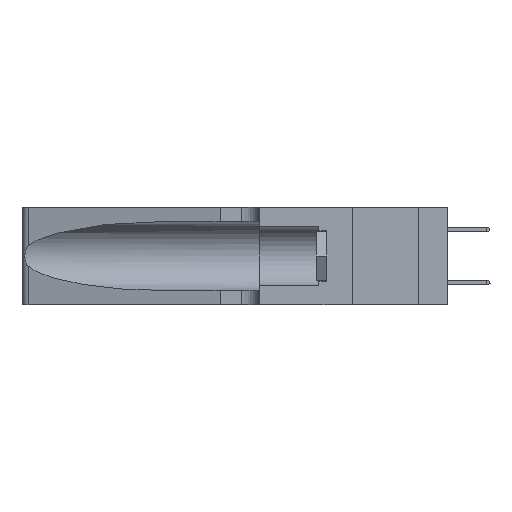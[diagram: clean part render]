
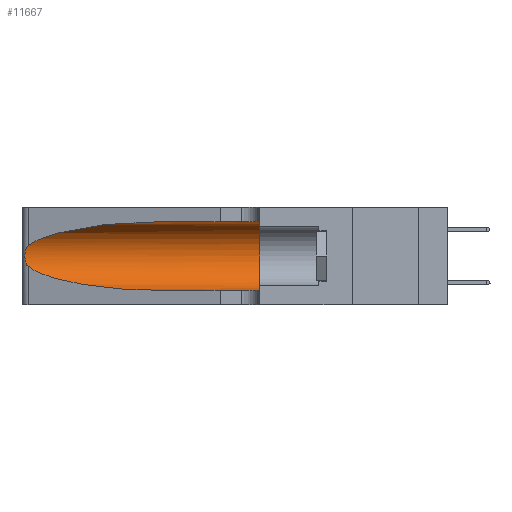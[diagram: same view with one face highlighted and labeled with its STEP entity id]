
A CAD part, left-side view. The second image highlights one B-rep face of the part: STEP entity #11667.
In plain terms, the highlighted cylindrical face has radius 3.308 mm (diameter 6.617 mm), a partial arc.
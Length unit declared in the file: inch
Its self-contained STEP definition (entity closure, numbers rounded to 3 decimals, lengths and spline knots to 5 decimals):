
#311 = VERTEX_POINT ( 'NONE', #428 ) ;
#428 = CARTESIAN_POINT ( 'NONE',  ( 0.1305, 0.72297, 0.05475 ) ) ;
#748 = CARTESIAN_POINT ( 'NONE',  ( 0.26017, 1.23833, 0.17102 ) ) ;
#1213 =( BOUNDED_CURVE ( )  B_SPLINE_CURVE ( 3, ( #29849, #4670, #22316, #2361 ),
 .UNSPECIFIED., .F., .T. ) 
 B_SPLINE_CURVE_WITH_KNOTS ( ( 4, 4 ),
 ( 1.5708, 2.84003 ),
 .UNSPECIFIED. ) 
 CURVE ( )  GEOMETRIC_REPRESENTATION_ITEM ( )  RATIONAL_B_SPLINE_CURVE ( ( 1., 0.87, 0.87, 1. ) ) 
 REPRESENTATION_ITEM ( '' )  );
#1276 = EDGE_CURVE ( 'NONE', #22835, #1857, #1213, .T. ) ;
#1351 = CYLINDRICAL_SURFACE ( 'NONE', #23014, 0.13025 ) ;
#1857 = VERTEX_POINT ( 'NONE', #15176 ) ;
#2094 = CIRCLE ( 'NONE', #8127, 0.13025 ) ;
#2361 = CARTESIAN_POINT ( 'NONE',  ( 0.25487, 1.22718, 0.22369 ) ) ;
#2456 = DIRECTION ( 'NONE',  ( 0., -1., 0. ) ) ;
#2646 = EDGE_CURVE ( 'NONE', #1857, #17677, #9089, .T. ) ;
#3270 = CARTESIAN_POINT ( 'NONE',  ( 0.26075, 1.23896, 0.19203 ) ) ;
#3482 = CARTESIAN_POINT ( 'NONE',  ( 0.25555, 1.22994, 0.2215 ) ) ;
#4023 = DIRECTION ( 'NONE',  ( 0., 1., 0. ) ) ;
#4670 = CARTESIAN_POINT ( 'NONE',  ( 0.18966, 0.96281, 0.31525 ) ) ;
#5170 = CARTESIAN_POINT ( 'NONE',  ( 0.18966, 0.96281, 0.05475 ) ) ;
#5290 = ORIENTED_EDGE ( 'NONE', *, *, #2646, .T. ) ;
#5950 = EDGE_CURVE ( 'NONE', #30631, #10290, #2094, .T. ) ;
#6088 = EDGE_CURVE ( 'NONE', #22835, #30631, #28123, .T. ) ;
#6875 = FACE_OUTER_BOUND ( 'NONE', #13525, .T. ) ;
#7807 = EDGE_CURVE ( 'NONE', #17677, #311, #10099, .T. ) ;
#7984 = ORIENTED_EDGE ( 'NONE', *, *, #5950, .F. ) ;
#8127 = AXIS2_PLACEMENT_3D ( 'NONE', #16268, #4023, #18768 ) ;
#8325 = CARTESIAN_POINT ( 'NONE',  ( 0.25487, 1.22718, 0.14631 ) ) ;
#8363 = VECTOR ( 'NONE', #23305, 39.37008 ) ;
#8463 = CARTESIAN_POINT ( 'NONE',  ( 0.25487, 1.22718, 0.14631 ) ) ;
#8469 = ORIENTED_EDGE ( 'NONE', *, *, #26718, .T. ) ;
#9089 = B_SPLINE_CURVE_WITH_KNOTS ( 'NONE', 3,
 ( #13322, #3482, #10686, #26232, #13214, #23803, #3270, #31138, #748, #21122, #23702, #11120, #18343, #8463 ),
 .UNSPECIFIED., .F., .F.,
 ( 4, 2, 2, 2, 2, 2, 4 ),
 ( 0., 0.00027, 0.00053, 0.00107, 0.0016, 0.00187, 0.00214 ),
 .UNSPECIFIED. ) ;
#10099 =( BOUNDED_CURVE ( )  B_SPLINE_CURVE ( 3, ( #19806, #24949, #5170, #15307 ),
 .UNSPECIFIED., .F., .F. ) 
 B_SPLINE_CURVE_WITH_KNOTS ( ( 4, 4 ),
 ( 3.44316, 4.71239 ),
 .UNSPECIFIED. ) 
 CURVE ( )  GEOMETRIC_REPRESENTATION_ITEM ( )  RATIONAL_B_SPLINE_CURVE ( ( 1., 0.87, 0.87, 1. ) ) 
 REPRESENTATION_ITEM ( '' )  );
#10290 = VERTEX_POINT ( 'NONE', #22387 ) ;
#10686 = CARTESIAN_POINT ( 'NONE',  ( 0.25639, 1.23184, 0.21858 ) ) ;
#11120 = CARTESIAN_POINT ( 'NONE',  ( 0.25639, 1.23186, 0.15144 ) ) ;
#11667 = ADVANCED_FACE ( 'NONE', ( #6875 ), #1351, .F. ) ;
#13214 = CARTESIAN_POINT ( 'NONE',  ( 0.25854, 1.2359, 0.20912 ) ) ;
#13322 = CARTESIAN_POINT ( 'NONE',  ( 0.25487, 1.22718, 0.22369 ) ) ;
#13525 = EDGE_LOOP ( 'NONE', ( #13726, #5290, #20700, #8469, #7984, #23280 ) ) ;
#13726 = ORIENTED_EDGE ( 'NONE', *, *, #1276, .T. ) ;
#15176 = CARTESIAN_POINT ( 'NONE',  ( 0.25487, 1.22718, 0.22369 ) ) ;
#15307 = CARTESIAN_POINT ( 'NONE',  ( 0.1305, 0.72297, 0.05475 ) ) ;
#16268 = CARTESIAN_POINT ( 'NONE',  ( 0.1305, 0.35, 0.185 ) ) ;
#17677 = VERTEX_POINT ( 'NONE', #8325 ) ;
#18215 = VECTOR ( 'NONE', #2456, 39.37008 ) ;
#18343 = CARTESIAN_POINT ( 'NONE',  ( 0.25555, 1.22993, 0.14849 ) ) ;
#18378 = CARTESIAN_POINT ( 'NONE',  ( 0.1305, 1.61858, 0.31525 ) ) ;
#18645 = DIRECTION ( 'NONE',  ( 0., 0., -1. ) ) ;
#18768 = DIRECTION ( 'NONE',  ( 0., 0., 1. ) ) ;
#19806 = CARTESIAN_POINT ( 'NONE',  ( 0.25487, 1.22718, 0.14631 ) ) ;
#20700 = ORIENTED_EDGE ( 'NONE', *, *, #7807, .T. ) ;
#21122 = CARTESIAN_POINT ( 'NONE',  ( 0.25856, 1.23593, 0.16098 ) ) ;
#21441 = DIRECTION ( 'NONE',  ( 0., -1., 0. ) ) ;
#22316 = CARTESIAN_POINT ( 'NONE',  ( 0.2373, 1.15595, 0.28018 ) ) ;
#22387 = CARTESIAN_POINT ( 'NONE',  ( 0.1305, 0.35, 0.05475 ) ) ;
#22586 = CARTESIAN_POINT ( 'NONE',  ( 0.1305, 0.72297, 0.31525 ) ) ;
#22753 = CARTESIAN_POINT ( 'NONE',  ( 0.1305, 1.61858, 0.05475 ) ) ;
#22835 = VERTEX_POINT ( 'NONE', #22586 ) ;
#23014 = AXIS2_PLACEMENT_3D ( 'NONE', #29095, #21441, #18645 ) ;
#23280 = ORIENTED_EDGE ( 'NONE', *, *, #6088, .F. ) ;
#23305 = DIRECTION ( 'NONE',  ( 0., -1., 0. ) ) ;
#23702 = CARTESIAN_POINT ( 'NONE',  ( 0.25789, 1.23486, 0.15765 ) ) ;
#23803 = CARTESIAN_POINT ( 'NONE',  ( 0.26018, 1.23835, 0.19895 ) ) ;
#24949 = CARTESIAN_POINT ( 'NONE',  ( 0.2373, 1.15595, 0.08982 ) ) ;
#26232 = CARTESIAN_POINT ( 'NONE',  ( 0.25787, 1.23484, 0.2124 ) ) ;
#26612 = CARTESIAN_POINT ( 'NONE',  ( 0.1305, 0.35, 0.31525 ) ) ;
#26718 = EDGE_CURVE ( 'NONE', #311, #10290, #28186, .T. ) ;
#28123 = LINE ( 'NONE', #18378, #8363 ) ;
#28186 = LINE ( 'NONE', #22753, #18215 ) ;
#29095 = CARTESIAN_POINT ( 'NONE',  ( 0.1305, 1.61858, 0.185 ) ) ;
#29849 = CARTESIAN_POINT ( 'NONE',  ( 0.1305, 0.72297, 0.31525 ) ) ;
#30631 = VERTEX_POINT ( 'NONE', #26612 ) ;
#31138 = CARTESIAN_POINT ( 'NONE',  ( 0.26075, 1.23896, 0.178 ) ) ;
